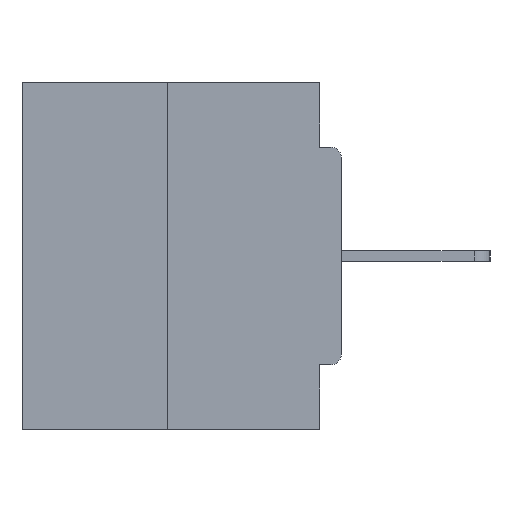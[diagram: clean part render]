
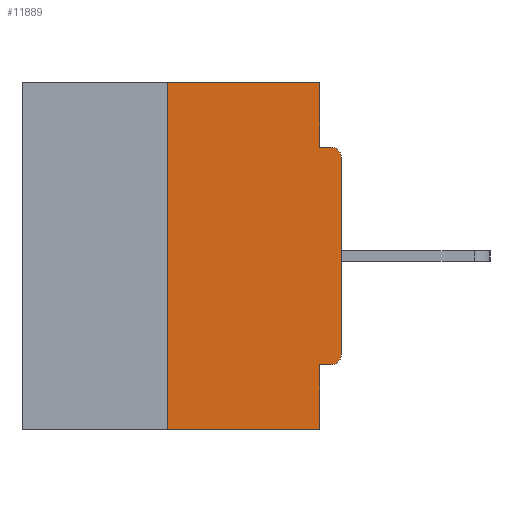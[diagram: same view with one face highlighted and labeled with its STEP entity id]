
A CAD part, left-side view. The second image highlights one B-rep face of the part: STEP entity #11889.
In plain terms, the highlighted planar face has unit normal (-1, 0, 0).
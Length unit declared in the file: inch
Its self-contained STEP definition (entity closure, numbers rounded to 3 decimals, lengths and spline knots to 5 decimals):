
#1204 = LINE ( 'NONE', #23133, #23918 ) ;
#1490 = DIRECTION ( 'NONE',  ( 0., -1., 0. ) ) ;
#1499 = CARTESIAN_POINT ( 'NONE',  ( 0., 0.25, 0. ) ) ;
#1688 = DIRECTION ( 'NONE',  ( 1., 0., 0. ) ) ;
#1970 = VECTOR ( 'NONE', #9544, 39.37008 ) ;
#3194 = CARTESIAN_POINT ( 'NONE',  ( 0., 0.031, -0.5 ) ) ;
#3988 = LINE ( 'NONE', #31482, #1970 ) ;
#4015 = ORIENTED_EDGE ( 'NONE', *, *, #17494, .F. ) ;
#4026 = PLANE ( 'NONE',  #15396 ) ;
#4079 = DIRECTION ( 'NONE',  ( 0., 0., 1. ) ) ;
#4113 = CARTESIAN_POINT ( 'NONE',  ( 0., 0.015, -0.1085 ) ) ;
#4188 = CARTESIAN_POINT ( 'NONE',  ( 0., 0.46, 0. ) ) ;
#4395 = DIRECTION ( 'NONE',  ( 0., 0., -1. ) ) ;
#4496 = VERTEX_POINT ( 'NONE', #31587 ) ;
#4636 = VERTEX_POINT ( 'NONE', #20988 ) ;
#4686 = CARTESIAN_POINT ( 'NONE',  ( 0., 0.031, 0. ) ) ;
#4909 = CARTESIAN_POINT ( 'NONE',  ( 0., 0., 0. ) ) ;
#5656 = DIRECTION ( 'NONE',  ( 0., -1., 0. ) ) ;
#6064 = CARTESIAN_POINT ( 'NONE',  ( 0., 0.46, 0. ) ) ;
#6450 = ORIENTED_EDGE ( 'NONE', *, *, #10034, .T. ) ;
#6730 = VERTEX_POINT ( 'NONE', #11756 ) ;
#6883 = LINE ( 'NONE', #4188, #7215 ) ;
#7215 = VECTOR ( 'NONE', #1490, 39.37008 ) ;
#7591 = EDGE_LOOP ( 'NONE', ( #7956, #28737, #6450, #33150, #10437, #10618, #12528, #21091, #4015, #17263 ) ) ;
#7956 = ORIENTED_EDGE ( 'NONE', *, *, #31187, .F. ) ;
#9057 = VERTEX_POINT ( 'NONE', #1499 ) ;
#9544 = DIRECTION ( 'NONE',  ( 0., 1., 0. ) ) ;
#9551 = VERTEX_POINT ( 'NONE', #4686 ) ;
#10034 = EDGE_CURVE ( 'NONE', #28641, #22623, #27059, .T. ) ;
#10125 = DIRECTION ( 'NONE',  ( 0., 0., -1. ) ) ;
#10437 = ORIENTED_EDGE ( 'NONE', *, *, #20623, .F. ) ;
#10618 = ORIENTED_EDGE ( 'NONE', *, *, #11876, .T. ) ;
#10645 = LINE ( 'NONE', #29346, #34013 ) ;
#11756 = CARTESIAN_POINT ( 'NONE',  ( 0., 0.031, -0.0935 ) ) ;
#11876 = EDGE_CURVE ( 'NONE', #24358, #4636, #13675, .T. ) ;
#11889 = ADVANCED_FACE ( 'NONE', ( #34401 ), #4026, .F. ) ;
#12044 = LINE ( 'NONE', #33629, #21955 ) ;
#12199 = DIRECTION ( 'NONE',  ( 0., 0., -1. ) ) ;
#12299 = DIRECTION ( 'NONE',  ( 0., 0., -1. ) ) ;
#12528 = ORIENTED_EDGE ( 'NONE', *, *, #26190, .T. ) ;
#13675 = CIRCLE ( 'NONE', #32588, 0.015 ) ;
#14760 = DIRECTION ( 'NONE',  ( 0., -1., 0. ) ) ;
#15396 = AXIS2_PLACEMENT_3D ( 'NONE', #6064, #1688, #12299 ) ;
#15878 = DIRECTION ( 'NONE',  ( 0., 0., 1. ) ) ;
#17263 = ORIENTED_EDGE ( 'NONE', *, *, #28201, .F. ) ;
#17494 = EDGE_CURVE ( 'NONE', #6730, #30562, #12044, .T. ) ;
#18006 = CARTESIAN_POINT ( 'NONE',  ( 0., 0.25, -0.5 ) ) ;
#18693 = CARTESIAN_POINT ( 'NONE',  ( 0., 0.031, -0.5 ) ) ;
#19059 = EDGE_CURVE ( 'NONE', #4496, #22623, #30179, .T. ) ;
#19400 = DIRECTION ( 'NONE',  ( 0., 0., -1. ) ) ;
#20389 = CARTESIAN_POINT ( 'NONE',  ( 0., 0.015, -0.3915 ) ) ;
#20485 = CARTESIAN_POINT ( 'NONE',  ( 0., 0., -0.1085 ) ) ;
#20623 = EDGE_CURVE ( 'NONE', #24358, #4496, #3988, .T. ) ;
#20988 = CARTESIAN_POINT ( 'NONE',  ( 0., 0., -0.3915 ) ) ;
#21091 = ORIENTED_EDGE ( 'NONE', *, *, #27152, .T. ) ;
#21273 = LINE ( 'NONE', #4909, #26889 ) ;
#21955 = VECTOR ( 'NONE', #14760, 39.37008 ) ;
#22381 = VERTEX_POINT ( 'NONE', #20485 ) ;
#22623 = VERTEX_POINT ( 'NONE', #3194 ) ;
#22776 = EDGE_CURVE ( 'NONE', #28641, #9057, #1204, .T. ) ;
#23133 = CARTESIAN_POINT ( 'NONE',  ( 0., 0.25, 0. ) ) ;
#23703 = DIRECTION ( 'NONE',  ( -1., 0., 0. ) ) ;
#23795 = DIRECTION ( 'NONE',  ( -1., 0., 0. ) ) ;
#23918 = VECTOR ( 'NONE', #4079, 39.37008 ) ;
#24358 = VERTEX_POINT ( 'NONE', #31371 ) ;
#25913 = AXIS2_PLACEMENT_3D ( 'NONE', #4113, #23703, #12199 ) ;
#26190 = EDGE_CURVE ( 'NONE', #4636, #22381, #21273, .T. ) ;
#26889 = VECTOR ( 'NONE', #15878, 39.37008 ) ;
#27059 = LINE ( 'NONE', #32971, #31302 ) ;
#27152 = EDGE_CURVE ( 'NONE', #22381, #30562, #32779, .T. ) ;
#27203 = CARTESIAN_POINT ( 'NONE',  ( 0., 0.015, -0.0935 ) ) ;
#28201 = EDGE_CURVE ( 'NONE', #9551, #6730, #10645, .T. ) ;
#28641 = VERTEX_POINT ( 'NONE', #18006 ) ;
#28737 = ORIENTED_EDGE ( 'NONE', *, *, #22776, .F. ) ;
#29346 = CARTESIAN_POINT ( 'NONE',  ( 0., 0.031, 0. ) ) ;
#30179 = LINE ( 'NONE', #18693, #30656 ) ;
#30562 = VERTEX_POINT ( 'NONE', #27203 ) ;
#30656 = VECTOR ( 'NONE', #19400, 39.37008 ) ;
#31187 = EDGE_CURVE ( 'NONE', #9057, #9551, #6883, .T. ) ;
#31302 = VECTOR ( 'NONE', #5656, 39.37008 ) ;
#31371 = CARTESIAN_POINT ( 'NONE',  ( 0., 0.015, -0.4065 ) ) ;
#31482 = CARTESIAN_POINT ( 'NONE',  ( 0., 0., -0.4065 ) ) ;
#31587 = CARTESIAN_POINT ( 'NONE',  ( 0., 0.031, -0.4065 ) ) ;
#32588 = AXIS2_PLACEMENT_3D ( 'NONE', #20389, #23795, #10125 ) ;
#32779 = CIRCLE ( 'NONE', #25913, 0.015 ) ;
#32971 = CARTESIAN_POINT ( 'NONE',  ( 0., 0.46, -0.5 ) ) ;
#33150 = ORIENTED_EDGE ( 'NONE', *, *, #19059, .F. ) ;
#33629 = CARTESIAN_POINT ( 'NONE',  ( 0., 0., -0.0935 ) ) ;
#34013 = VECTOR ( 'NONE', #4395, 39.37008 ) ;
#34401 = FACE_OUTER_BOUND ( 'NONE', #7591, .T. ) ;
